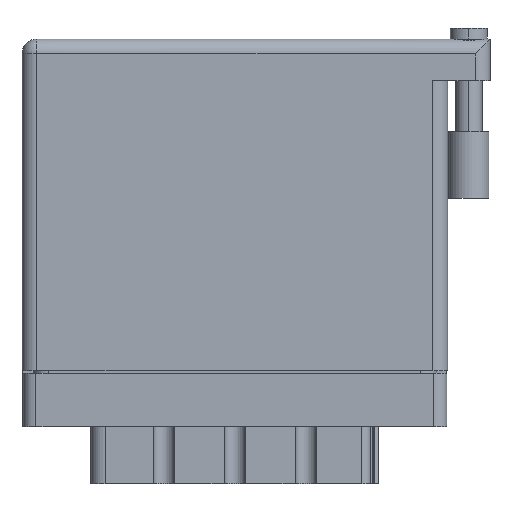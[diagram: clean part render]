
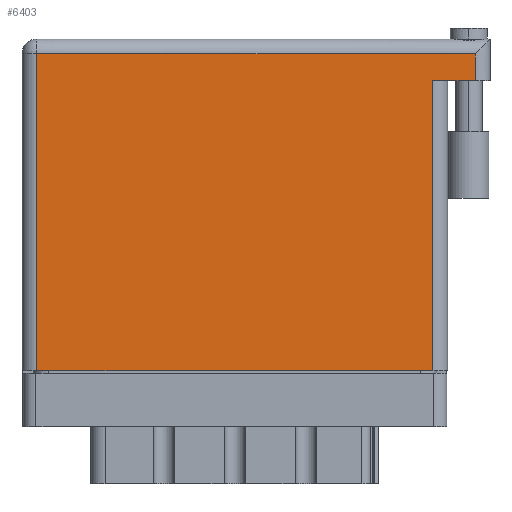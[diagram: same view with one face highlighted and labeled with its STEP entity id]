
A CAD part, front view. The second image highlights one B-rep face of the part: STEP entity #6403.
In plain terms, the highlighted face is planar.
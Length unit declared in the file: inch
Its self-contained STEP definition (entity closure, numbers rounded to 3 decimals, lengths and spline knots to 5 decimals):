
#364 = VERTEX_POINT ( 'NONE', #30283 ) ;
#405 = VERTEX_POINT ( 'NONE', #24202 ) ;
#1735 = VERTEX_POINT ( 'NONE', #23019 ) ;
#1875 = LINE ( 'NONE', #3406, #19729 ) ;
#2101 = LINE ( 'NONE', #22472, #13530 ) ;
#2525 = EDGE_CURVE ( 'NONE', #38848, #40177, #19073, .T. ) ;
#2657 = ORIENTED_EDGE ( 'NONE', *, *, #38216, .T. ) ;
#3350 = DIRECTION ( 'NONE',  ( -1., 0., 0. ) ) ;
#3406 = CARTESIAN_POINT ( 'NONE',  ( 0., 0., 0. ) ) ;
#4628 = VECTOR ( 'NONE', #38772, 39.37008 ) ;
#6403 = ADVANCED_FACE ( 'NONE', ( #9497 ), #10023, .F. ) ;
#7362 = ORIENTED_EDGE ( 'NONE', *, *, #21812, .T. ) ;
#7799 = ORIENTED_EDGE ( 'NONE', *, *, #8500, .T. ) ;
#8206 = VECTOR ( 'NONE', #18816, 39.37008 ) ;
#8500 = EDGE_CURVE ( 'NONE', #364, #405, #1875, .T. ) ;
#9175 = EDGE_LOOP ( 'NONE', ( #7799, #7362, #20791, #18274, #25939, #2657 ) ) ;
#9497 = FACE_OUTER_BOUND ( 'NONE', #9175, .T. ) ;
#10023 = PLANE ( 'NONE',  #31005 ) ;
#10969 = CARTESIAN_POINT ( 'NONE',  ( 0., 1.496, 0. ) ) ;
#12821 = EDGE_CURVE ( 'NONE', #38848, #23953, #2101, .T. ) ;
#12875 = VECTOR ( 'NONE', #23718, 39.37008 ) ;
#13530 = VECTOR ( 'NONE', #34935, 39.37008 ) ;
#13701 = CARTESIAN_POINT ( 'NONE',  ( 2.138, 1.369, 0. ) ) ;
#16647 = CARTESIAN_POINT ( 'NONE',  ( 0.07, 0., 0. ) ) ;
#18274 = ORIENTED_EDGE ( 'NONE', *, *, #12821, .T. ) ;
#18816 = DIRECTION ( 'NONE',  ( -1., 0., 0. ) ) ;
#19073 = LINE ( 'NONE', #34597, #8206 ) ;
#19082 = DIRECTION ( 'NONE',  ( 1., 0., 0. ) ) ;
#19729 = VECTOR ( 'NONE', #19082, 39.37008 ) ;
#20323 = LINE ( 'NONE', #10969, #12875 ) ;
#20791 = ORIENTED_EDGE ( 'NONE', *, *, #2525, .F. ) ;
#21812 = EDGE_CURVE ( 'NONE', #405, #40177, #38330, .T. ) ;
#22472 = CARTESIAN_POINT ( 'NONE',  ( 2.138, 1.566, 0. ) ) ;
#23019 = CARTESIAN_POINT ( 'NONE',  ( 0.07, 1.496, 0. ) ) ;
#23718 = DIRECTION ( 'NONE',  ( -1., 0., 0. ) ) ;
#23953 = VERTEX_POINT ( 'NONE', #30440 ) ;
#24062 = LINE ( 'NONE', #16647, #35420 ) ;
#24202 = CARTESIAN_POINT ( 'NONE',  ( 1.938, 0., 0. ) ) ;
#25810 = DIRECTION ( 'NONE',  ( 0., 0., -1. ) ) ;
#25939 = ORIENTED_EDGE ( 'NONE', *, *, #28332, .T. ) ;
#26722 = CARTESIAN_POINT ( 'NONE',  ( 1.938, 1.369, 0. ) ) ;
#28332 = EDGE_CURVE ( 'NONE', #23953, #1735, #20323, .T. ) ;
#29793 = DIRECTION ( 'NONE',  ( 0., -1., 0. ) ) ;
#30283 = CARTESIAN_POINT ( 'NONE',  ( 0.07, 0., 0. ) ) ;
#30440 = CARTESIAN_POINT ( 'NONE',  ( 2.138, 1.496, 0. ) ) ;
#31005 = AXIS2_PLACEMENT_3D ( 'NONE', #38398, #25810, #3350 ) ;
#34597 = CARTESIAN_POINT ( 'NONE',  ( 2.208, 1.369, 0. ) ) ;
#34935 = DIRECTION ( 'NONE',  ( 0., 1., 0. ) ) ;
#35420 = VECTOR ( 'NONE', #29793, 39.37008 ) ;
#35599 = CARTESIAN_POINT ( 'NONE',  ( 1.938, 1.369, 0. ) ) ;
#38216 = EDGE_CURVE ( 'NONE', #1735, #364, #24062, .T. ) ;
#38330 = LINE ( 'NONE', #35599, #4628 ) ;
#38398 = CARTESIAN_POINT ( 'NONE',  ( 0., 1.566, 0. ) ) ;
#38772 = DIRECTION ( 'NONE',  ( 0., 1., 0. ) ) ;
#38848 = VERTEX_POINT ( 'NONE', #13701 ) ;
#40177 = VERTEX_POINT ( 'NONE', #26722 ) ;
